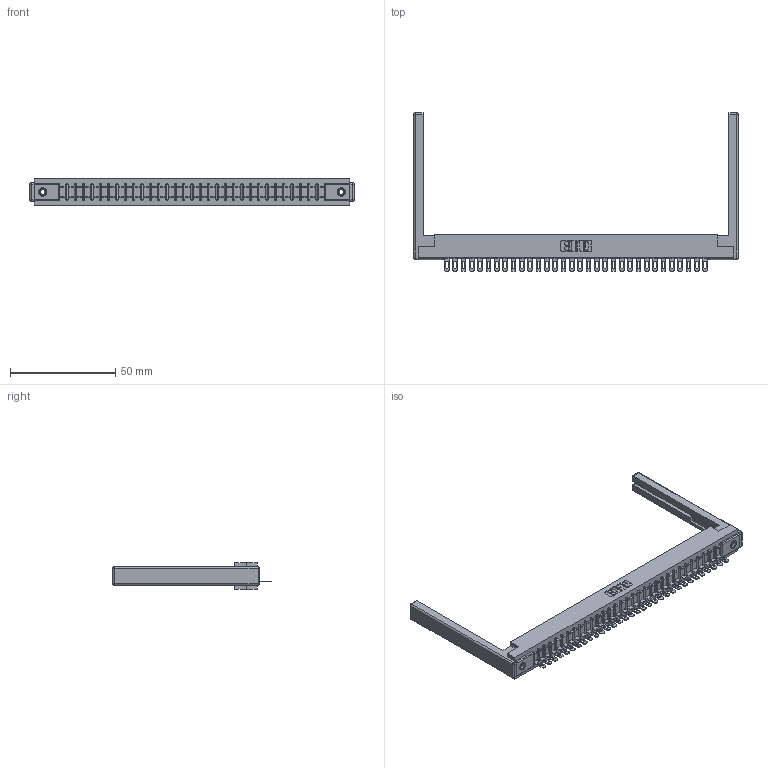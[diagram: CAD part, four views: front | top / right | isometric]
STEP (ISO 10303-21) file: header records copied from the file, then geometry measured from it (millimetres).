
FILE_DESCRIPTION (( 'STEP AP203' ), '1' );
FILE_NAME ('307-032-401-168.STEP', '2020-09-28T16:22:13', ( '' ), ( '' ), 'SwSTEP 2.0', 'SolidWorks 2020', '' );
FILE_SCHEMA (( 'CONFIG_CONTROL_DESIGN' ));
Length unit declared in the file: inch
Products named in the file (5): 345-250-001_345-250-001-102; 307-290-002_501; 307-220-068; 307 Part_.156 Dia Mounting Holes; 307-032-401-168
Assembly tree (37 placements, depth 2):
  307-032-401-168
    307 Part_.156 Dia Mounting Holes
    307-290-002_501  x32
    307-220-068  x2
    345-250-001_345-250-001-102  x2
Bounding box: 154.23 x 75.39 x 12.7 mm (x, y, z)
Volume: 20835.3 mm3; surface area: 24651.6 mm2
Topology: 37 solids, 37 shells, 2737 faces, 8329 edges, 5442 vertices
Faces by surface type: plane 1566, cylinder 1081, sphere 74, cone 12, torus 4
Entity records: 32219 total; most frequent: CARTESIAN_POINT 5397, ORIENTED_EDGE 5376, DIRECTION 5270, EDGE_CURVE 2688, LINE 2048, VECTOR 2048, VERTEX_POINT 1738, AXIS2_PLACEMENT_3D 1611
